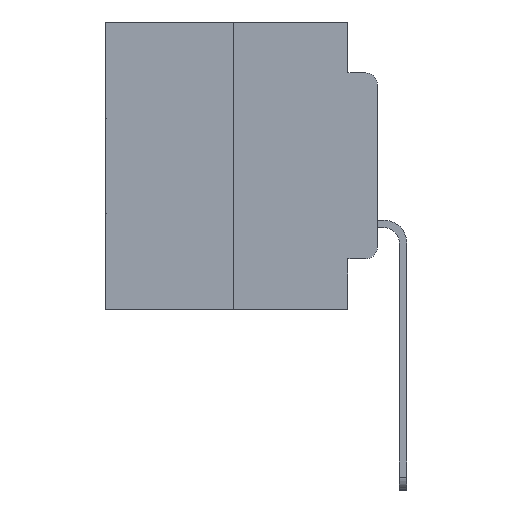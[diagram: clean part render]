
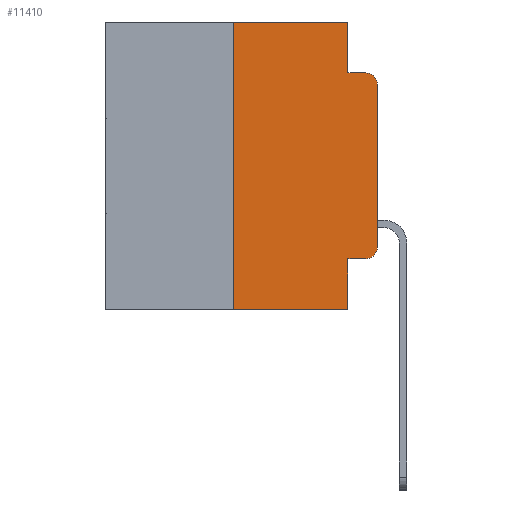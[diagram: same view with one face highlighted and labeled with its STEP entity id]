
A CAD part, left-side view. The second image highlights one B-rep face of the part: STEP entity #11410.
In plain terms, the highlighted planar face has unit normal (-1, 0, 0).
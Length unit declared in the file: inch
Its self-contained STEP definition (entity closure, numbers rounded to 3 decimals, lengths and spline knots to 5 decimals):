
#172 = EDGE_CURVE ( 'NONE', #27359, #2314, #7260, .T. ) ;
#261 = CARTESIAN_POINT ( 'NONE',  ( 0., 0.051, 0. ) ) ;
#948 = VERTEX_POINT ( 'NONE', #21680 ) ;
#1230 = AXIS2_PLACEMENT_3D ( 'NONE', #19194, #19366, #10756 ) ;
#1331 = ORIENTED_EDGE ( 'NONE', *, *, #23205, .F. ) ;
#1657 = EDGE_LOOP ( 'NONE', ( #19704, #17740, #1331, #12440, #2798, #16544, #3049, #6194, #23755, #26934 ) ) ;
#1993 = EDGE_CURVE ( 'NONE', #19376, #23673, #5794, .T. ) ;
#2314 = VERTEX_POINT ( 'NONE', #11710 ) ;
#2594 = CARTESIAN_POINT ( 'NONE',  ( 0., 0.473, 0. ) ) ;
#2798 = ORIENTED_EDGE ( 'NONE', *, *, #3876, .F. ) ;
#3049 = ORIENTED_EDGE ( 'NONE', *, *, #14505, .T. ) ;
#3876 = EDGE_CURVE ( 'NONE', #948, #20563, #19961, .T. ) ;
#3989 = VERTEX_POINT ( 'NONE', #17903 ) ;
#4333 = CARTESIAN_POINT ( 'NONE',  ( 0., 0.473, 0. ) ) ;
#4489 = CARTESIAN_POINT ( 'NONE',  ( 0., 0.051, -0.4115 ) ) ;
#4593 = DIRECTION ( 'NONE',  ( 0., -1., 0. ) ) ;
#4676 = DIRECTION ( 'NONE',  ( 0., 0., -1. ) ) ;
#5104 = VECTOR ( 'NONE', #4676, 39.37008 ) ;
#5146 = FACE_OUTER_BOUND ( 'NONE', #1657, .T. ) ;
#5382 = CARTESIAN_POINT ( 'NONE',  ( 0., 0.051, -0.4115 ) ) ;
#5794 = LINE ( 'NONE', #261, #5104 ) ;
#6194 = ORIENTED_EDGE ( 'NONE', *, *, #1993, .F. ) ;
#6771 = CARTESIAN_POINT ( 'NONE',  ( 0., 0., -0.3915 ) ) ;
#6772 = CARTESIAN_POINT ( 'NONE',  ( 0., 0.25, -0.5 ) ) ;
#6922 = CIRCLE ( 'NONE', #1230, 0.02 ) ;
#7020 = VERTEX_POINT ( 'NONE', #6772 ) ;
#7092 = EDGE_CURVE ( 'NONE', #7020, #948, #12292, .T. ) ;
#7206 = LINE ( 'NONE', #9977, #20439 ) ;
#7260 = LINE ( 'NONE', #8117, #11011 ) ;
#7378 = VERTEX_POINT ( 'NONE', #11619 ) ;
#7548 = EDGE_CURVE ( 'NONE', #19376, #3989, #25177, .T. ) ;
#8117 = CARTESIAN_POINT ( 'NONE',  ( 0., 0., 0. ) ) ;
#8856 = CARTESIAN_POINT ( 'NONE',  ( 0., 0.25, 0. ) ) ;
#9035 = VERTEX_POINT ( 'NONE', #27260 ) ;
#9445 = CARTESIAN_POINT ( 'NONE',  ( 0., 0.051, -0.5 ) ) ;
#9977 = CARTESIAN_POINT ( 'NONE',  ( 0., 0.051, -0.0885 ) ) ;
#10619 = EDGE_CURVE ( 'NONE', #20563, #7378, #12689, .T. ) ;
#10756 = DIRECTION ( 'NONE',  ( 0., 0., -1. ) ) ;
#11011 = VECTOR ( 'NONE', #21379, 39.37008 ) ;
#11410 = ADVANCED_FACE ( 'NONE', ( #5146 ), #11620, .F. ) ;
#11619 = CARTESIAN_POINT ( 'NONE',  ( 0., 0.051, -0.0885 ) ) ;
#11620 = PLANE ( 'NONE',  #18691 ) ;
#11710 = CARTESIAN_POINT ( 'NONE',  ( 0., 0., -0.1085 ) ) ;
#12292 = LINE ( 'NONE', #8856, #15689 ) ;
#12440 = ORIENTED_EDGE ( 'NONE', *, *, #10619, .F. ) ;
#12442 = LINE ( 'NONE', #17143, #26676 ) ;
#12689 = LINE ( 'NONE', #14036, #17433 ) ;
#12833 = DIRECTION ( 'NONE',  ( 0., 0., 1. ) ) ;
#12914 = DIRECTION ( 'NONE',  ( 0., -1., 0. ) ) ;
#13085 = CARTESIAN_POINT ( 'NONE',  ( 0., 0.02, -0.3915 ) ) ;
#13329 = CARTESIAN_POINT ( 'NONE',  ( 0., 0.051, 0. ) ) ;
#14036 = CARTESIAN_POINT ( 'NONE',  ( 0., 0.051, 0. ) ) ;
#14505 = EDGE_CURVE ( 'NONE', #7020, #23673, #12442, .T. ) ;
#15210 = DIRECTION ( 'NONE',  ( -1., 0., 0. ) ) ;
#15242 = DIRECTION ( 'NONE',  ( 0., -1., 0. ) ) ;
#15441 = CIRCLE ( 'NONE', #23203, 0.02 ) ;
#15689 = VECTOR ( 'NONE', #12833, 39.37008 ) ;
#16544 = ORIENTED_EDGE ( 'NONE', *, *, #7092, .F. ) ;
#16944 = VECTOR ( 'NONE', #4593, 39.37008 ) ;
#17061 = VECTOR ( 'NONE', #15242, 39.37008 ) ;
#17143 = CARTESIAN_POINT ( 'NONE',  ( 0., 0.473, -0.5 ) ) ;
#17433 = VECTOR ( 'NONE', #22671, 39.37008 ) ;
#17740 = ORIENTED_EDGE ( 'NONE', *, *, #20430, .T. ) ;
#17903 = CARTESIAN_POINT ( 'NONE',  ( 0., 0.02, -0.4115 ) ) ;
#17977 = DIRECTION ( 'NONE',  ( 0., 0., -1. ) ) ;
#18691 = AXIS2_PLACEMENT_3D ( 'NONE', #2594, #26367, #17977 ) ;
#19194 = CARTESIAN_POINT ( 'NONE',  ( 0., 0.02, -0.1085 ) ) ;
#19366 = DIRECTION ( 'NONE',  ( -1., 0., 0. ) ) ;
#19376 = VERTEX_POINT ( 'NONE', #4489 ) ;
#19578 = DIRECTION ( 'NONE',  ( 0., 0., -1. ) ) ;
#19704 = ORIENTED_EDGE ( 'NONE', *, *, #172, .T. ) ;
#19807 = EDGE_CURVE ( 'NONE', #3989, #27359, #15441, .T. ) ;
#19961 = LINE ( 'NONE', #4333, #16944 ) ;
#20430 = EDGE_CURVE ( 'NONE', #2314, #9035, #6922, .T. ) ;
#20439 = VECTOR ( 'NONE', #27283, 39.37008 ) ;
#20563 = VERTEX_POINT ( 'NONE', #13329 ) ;
#21379 = DIRECTION ( 'NONE',  ( 0., 0., 1. ) ) ;
#21680 = CARTESIAN_POINT ( 'NONE',  ( 0., 0.25, 0. ) ) ;
#22671 = DIRECTION ( 'NONE',  ( 0., 0., -1. ) ) ;
#23203 = AXIS2_PLACEMENT_3D ( 'NONE', #13085, #15210, #19578 ) ;
#23205 = EDGE_CURVE ( 'NONE', #7378, #9035, #7206, .T. ) ;
#23673 = VERTEX_POINT ( 'NONE', #9445 ) ;
#23755 = ORIENTED_EDGE ( 'NONE', *, *, #7548, .T. ) ;
#25177 = LINE ( 'NONE', #5382, #17061 ) ;
#26367 = DIRECTION ( 'NONE',  ( 1., 0., 0. ) ) ;
#26676 = VECTOR ( 'NONE', #12914, 39.37008 ) ;
#26934 = ORIENTED_EDGE ( 'NONE', *, *, #19807, .T. ) ;
#27260 = CARTESIAN_POINT ( 'NONE',  ( 0., 0.02, -0.0885 ) ) ;
#27283 = DIRECTION ( 'NONE',  ( 0., -1., 0. ) ) ;
#27359 = VERTEX_POINT ( 'NONE', #6771 ) ;
